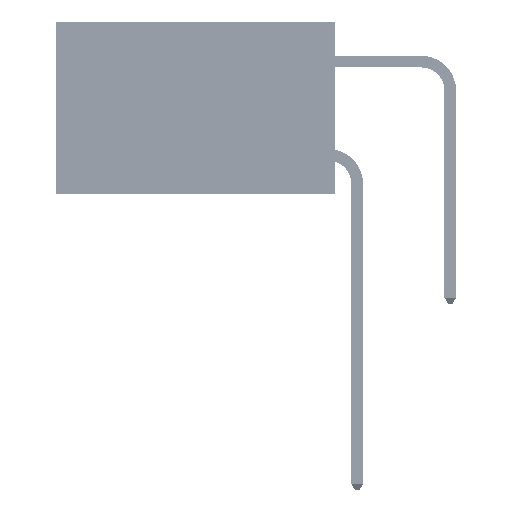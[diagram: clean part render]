
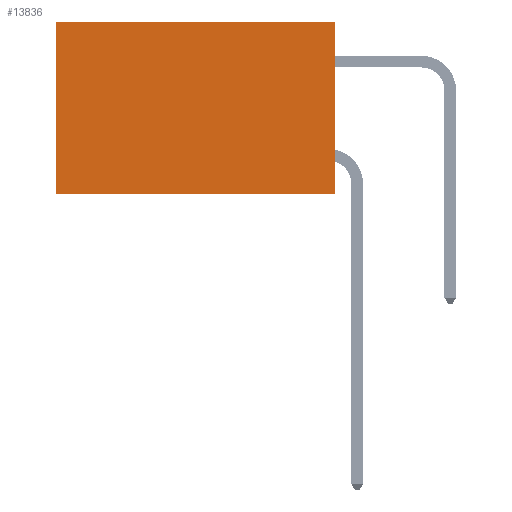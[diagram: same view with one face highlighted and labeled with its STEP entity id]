
A CAD part, left-side view. The second image highlights one B-rep face of the part: STEP entity #13836.
In plain terms, the highlighted planar face has unit normal (-1, 0, 0).
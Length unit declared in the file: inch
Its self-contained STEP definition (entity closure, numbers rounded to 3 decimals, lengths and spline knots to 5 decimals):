
#960 = AXIS2_PLACEMENT_3D ( 'NONE', #43754, #3061, #51698 ) ;
#1346 = ORIENTED_EDGE ( 'NONE', *, *, #19563, .F. ) ;
#2682 = CARTESIAN_POINT ( 'NONE',  ( 0.2875, 0.6, 0. ) ) ;
#3061 = DIRECTION ( 'NONE',  ( 1., 0., 0. ) ) ;
#3792 = VECTOR ( 'NONE', #51543, 39.37008 ) ;
#4034 = CARTESIAN_POINT ( 'NONE',  ( 0.2875, 0., -0.37 ) ) ;
#4387 = EDGE_CURVE ( 'NONE', #25956, #21587, #20946, .T. ) ;
#12745 = LINE ( 'NONE', #48013, #3792 ) ;
#13130 = VERTEX_POINT ( 'NONE', #18598 ) ;
#13836 = ADVANCED_FACE ( 'NONE', ( #46088 ), #43922, .F. ) ;
#14010 = LINE ( 'NONE', #20473, #45170 ) ;
#14709 = EDGE_LOOP ( 'NONE', ( #48455, #1346, #26901, #32883 ) ) ;
#16470 = EDGE_CURVE ( 'NONE', #13130, #25956, #12745, .T. ) ;
#18598 = CARTESIAN_POINT ( 'NONE',  ( 0.2875, 0., 0. ) ) ;
#19563 = EDGE_CURVE ( 'NONE', #47788, #21587, #39839, .T. ) ;
#20087 = VECTOR ( 'NONE', #20399, 39.37008 ) ;
#20294 = DIRECTION ( 'NONE',  ( 0., 0., -1. ) ) ;
#20399 = DIRECTION ( 'NONE',  ( 0., 1., 0. ) ) ;
#20473 = CARTESIAN_POINT ( 'NONE',  ( 0.2875, 0., 0. ) ) ;
#20946 = LINE ( 'NONE', #48350, #45779 ) ;
#21587 = VERTEX_POINT ( 'NONE', #25250 ) ;
#24377 = DIRECTION ( 'NONE',  ( 0., 0., -1. ) ) ;
#25250 = CARTESIAN_POINT ( 'NONE',  ( 0.2875, 0.6, -0.37 ) ) ;
#25956 = VERTEX_POINT ( 'NONE', #2682 ) ;
#26901 = ORIENTED_EDGE ( 'NONE', *, *, #29071, .F. ) ;
#29071 = EDGE_CURVE ( 'NONE', #13130, #47788, #14010, .T. ) ;
#32883 = ORIENTED_EDGE ( 'NONE', *, *, #16470, .T. ) ;
#39839 = LINE ( 'NONE', #4034, #20087 ) ;
#43754 = CARTESIAN_POINT ( 'NONE',  ( 0.2875, 0., 0. ) ) ;
#43922 = PLANE ( 'NONE',  #960 ) ;
#44291 = CARTESIAN_POINT ( 'NONE',  ( 0.2875, 0., -0.37 ) ) ;
#45170 = VECTOR ( 'NONE', #24377, 39.37008 ) ;
#45779 = VECTOR ( 'NONE', #20294, 39.37008 ) ;
#46088 = FACE_OUTER_BOUND ( 'NONE', #14709, .T. ) ;
#47788 = VERTEX_POINT ( 'NONE', #44291 ) ;
#48013 = CARTESIAN_POINT ( 'NONE',  ( 0.2875, 0., 0. ) ) ;
#48350 = CARTESIAN_POINT ( 'NONE',  ( 0.2875, 0.6, 0. ) ) ;
#48455 = ORIENTED_EDGE ( 'NONE', *, *, #4387, .T. ) ;
#51543 = DIRECTION ( 'NONE',  ( 0., 1., 0. ) ) ;
#51698 = DIRECTION ( 'NONE',  ( 0., 0., -1. ) ) ;
